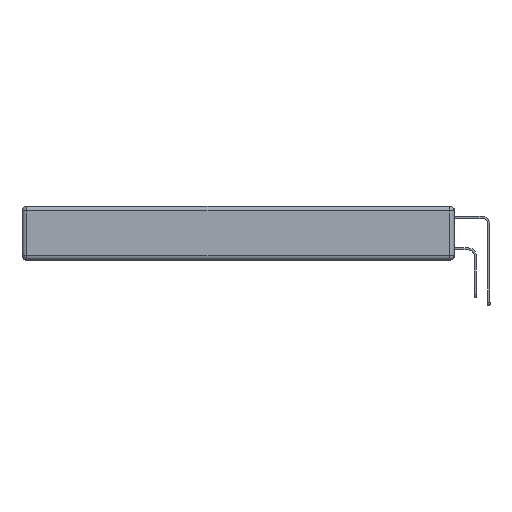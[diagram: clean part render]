
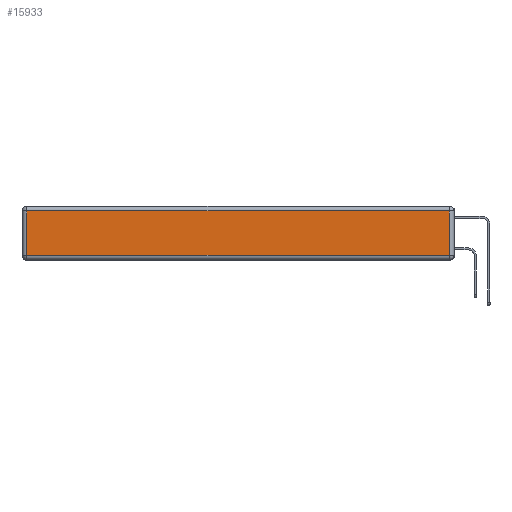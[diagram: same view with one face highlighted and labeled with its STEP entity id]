
A CAD part, left-side view. The second image highlights one B-rep face of the part: STEP entity #15933.
In plain terms, the highlighted planar face has unit normal (-1, 0, 0).
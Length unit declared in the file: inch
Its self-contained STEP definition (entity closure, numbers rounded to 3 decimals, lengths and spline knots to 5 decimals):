
#1209 = DIRECTION ( 'NONE',  ( 0., -1., 0. ) ) ;
#1482 = CARTESIAN_POINT ( 'NONE',  ( 0., 2.72, -0.03 ) ) ;
#4703 = EDGE_LOOP ( 'NONE', ( #21557, #15482, #12519, #13245 ) ) ;
#5037 = EDGE_CURVE ( 'NONE', #25210, #20744, #25863, .T. ) ;
#6598 = DIRECTION ( 'NONE',  ( 0., 0., 1. ) ) ;
#7409 = FACE_OUTER_BOUND ( 'NONE', #4703, .T. ) ;
#7550 = PLANE ( 'NONE',  #24148 ) ;
#7581 = CARTESIAN_POINT ( 'NONE',  ( 0., 0., -0.313 ) ) ;
#8437 = VECTOR ( 'NONE', #23611, 39.37008 ) ;
#8612 = VERTEX_POINT ( 'NONE', #15951 ) ;
#9208 = DIRECTION ( 'NONE',  ( 0., 0., -1. ) ) ;
#9449 = EDGE_CURVE ( 'NONE', #20744, #22040, #17023, .T. ) ;
#9813 = DIRECTION ( 'NONE',  ( 0., 0., 1. ) ) ;
#10689 = VECTOR ( 'NONE', #1209, 39.37008 ) ;
#11245 = VECTOR ( 'NONE', #9208, 39.37008 ) ;
#12519 = ORIENTED_EDGE ( 'NONE', *, *, #9449, .T. ) ;
#12951 = CARTESIAN_POINT ( 'NONE',  ( 0., 0.03, -0.03 ) ) ;
#13091 = CARTESIAN_POINT ( 'NONE',  ( 0., 0.03, -0.343 ) ) ;
#13245 = ORIENTED_EDGE ( 'NONE', *, *, #22787, .T. ) ;
#15395 = EDGE_CURVE ( 'NONE', #8612, #25210, #24731, .T. ) ;
#15482 = ORIENTED_EDGE ( 'NONE', *, *, #5037, .T. ) ;
#15816 = LINE ( 'NONE', #22254, #11245 ) ;
#15933 = ADVANCED_FACE ( 'NONE', ( #7409 ), #7550, .T. ) ;
#15951 = CARTESIAN_POINT ( 'NONE',  ( 0., 2.72, -0.313 ) ) ;
#15994 = CARTESIAN_POINT ( 'NONE',  ( 0., 0., -0.343 ) ) ;
#17023 = LINE ( 'NONE', #25444, #8437 ) ;
#19604 = CARTESIAN_POINT ( 'NONE',  ( 0., 0.03, -0.313 ) ) ;
#20744 = VERTEX_POINT ( 'NONE', #12951 ) ;
#21557 = ORIENTED_EDGE ( 'NONE', *, *, #15395, .T. ) ;
#22040 = VERTEX_POINT ( 'NONE', #1482 ) ;
#22254 = CARTESIAN_POINT ( 'NONE',  ( 0., 2.72, -0.343 ) ) ;
#22787 = EDGE_CURVE ( 'NONE', #22040, #8612, #15816, .T. ) ;
#23611 = DIRECTION ( 'NONE',  ( 0., 1., 0. ) ) ;
#24148 = AXIS2_PLACEMENT_3D ( 'NONE', #15994, #27079, #9813 ) ;
#24731 = LINE ( 'NONE', #7581, #10689 ) ;
#25210 = VERTEX_POINT ( 'NONE', #19604 ) ;
#25444 = CARTESIAN_POINT ( 'NONE',  ( 0., 2.75, -0.03 ) ) ;
#25863 = LINE ( 'NONE', #13091, #25896 ) ;
#25896 = VECTOR ( 'NONE', #6598, 39.37008 ) ;
#27079 = DIRECTION ( 'NONE',  ( -1., 0., 0. ) ) ;
